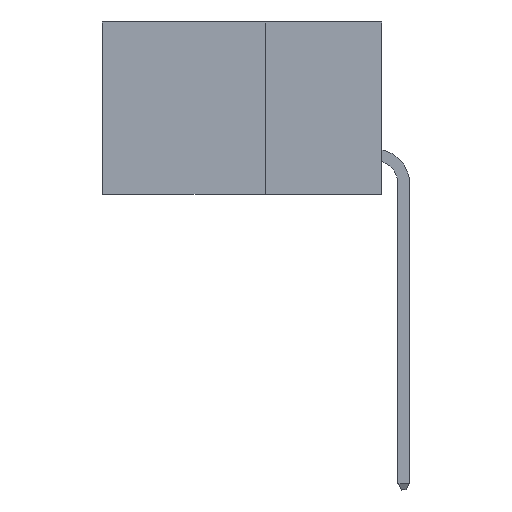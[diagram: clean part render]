
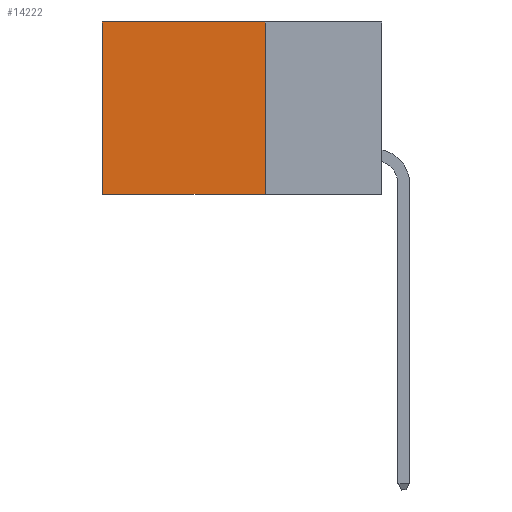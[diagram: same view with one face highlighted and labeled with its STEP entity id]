
A CAD part, left-side view. The second image highlights one B-rep face of the part: STEP entity #14222.
In plain terms, the highlighted planar face has unit normal (-1, 0, 0).
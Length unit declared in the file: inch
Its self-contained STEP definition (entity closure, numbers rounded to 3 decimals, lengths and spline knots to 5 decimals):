
#794 = DIRECTION ( 'NONE',  ( 0., 0., -1. ) ) ;
#1052 = LINE ( 'NONE', #19703, #11384 ) ;
#3965 = CARTESIAN_POINT ( 'NONE',  ( 0.2875, 0.25, -0.37 ) ) ;
#4769 = LINE ( 'NONE', #3965, #24544 ) ;
#5836 = EDGE_CURVE ( 'NONE', #21006, #19000, #1052, .T. ) ;
#6101 = DIRECTION ( 'NONE',  ( 0., 0., -1. ) ) ;
#6549 = ORIENTED_EDGE ( 'NONE', *, *, #20711, .T. ) ;
#7535 = CARTESIAN_POINT ( 'NONE',  ( 0.2875, 0.25, 0. ) ) ;
#8915 = LINE ( 'NONE', #22250, #16568 ) ;
#9349 = CARTESIAN_POINT ( 'NONE',  ( 0.2875, 0.6, 0. ) ) ;
#11384 = VECTOR ( 'NONE', #22034, 39.37008 ) ;
#13056 = EDGE_CURVE ( 'NONE', #21006, #24528, #28344, .T. ) ;
#13717 = VECTOR ( 'NONE', #794, 39.37008 ) ;
#14222 = ADVANCED_FACE ( 'NONE', ( #27948 ), #23143, .F. ) ;
#14983 = AXIS2_PLACEMENT_3D ( 'NONE', #25287, #30343, #27867 ) ;
#15336 = EDGE_CURVE ( 'NONE', #24528, #20908, #4769, .T. ) ;
#16568 = VECTOR ( 'NONE', #6101, 39.37008 ) ;
#17129 = ORIENTED_EDGE ( 'NONE', *, *, #15336, .F. ) ;
#18369 = ORIENTED_EDGE ( 'NONE', *, *, #5836, .T. ) ;
#19000 = VERTEX_POINT ( 'NONE', #9349 ) ;
#19703 = CARTESIAN_POINT ( 'NONE',  ( 0.2875, 0.25, 0. ) ) ;
#19872 = EDGE_LOOP ( 'NONE', ( #6549, #17129, #24192, #18369 ) ) ;
#20711 = EDGE_CURVE ( 'NONE', #19000, #20908, #8915, .T. ) ;
#20908 = VERTEX_POINT ( 'NONE', #27601 ) ;
#21006 = VERTEX_POINT ( 'NONE', #7535 ) ;
#21650 = CARTESIAN_POINT ( 'NONE',  ( 0.2875, 0.25, -0.37 ) ) ;
#22034 = DIRECTION ( 'NONE',  ( 0., 1., 0. ) ) ;
#22250 = CARTESIAN_POINT ( 'NONE',  ( 0.2875, 0.6, 0. ) ) ;
#23143 = PLANE ( 'NONE',  #14983 ) ;
#23986 = CARTESIAN_POINT ( 'NONE',  ( 0.2875, 0.25, 0. ) ) ;
#24192 = ORIENTED_EDGE ( 'NONE', *, *, #13056, .F. ) ;
#24528 = VERTEX_POINT ( 'NONE', #21650 ) ;
#24544 = VECTOR ( 'NONE', #29402, 39.37008 ) ;
#25287 = CARTESIAN_POINT ( 'NONE',  ( 0.2875, 0.25, 0. ) ) ;
#27601 = CARTESIAN_POINT ( 'NONE',  ( 0.2875, 0.6, -0.37 ) ) ;
#27867 = DIRECTION ( 'NONE',  ( 0., 0., -1. ) ) ;
#27948 = FACE_OUTER_BOUND ( 'NONE', #19872, .T. ) ;
#28344 = LINE ( 'NONE', #23986, #13717 ) ;
#29402 = DIRECTION ( 'NONE',  ( 0., 1., 0. ) ) ;
#30343 = DIRECTION ( 'NONE',  ( 1., 0., 0. ) ) ;
